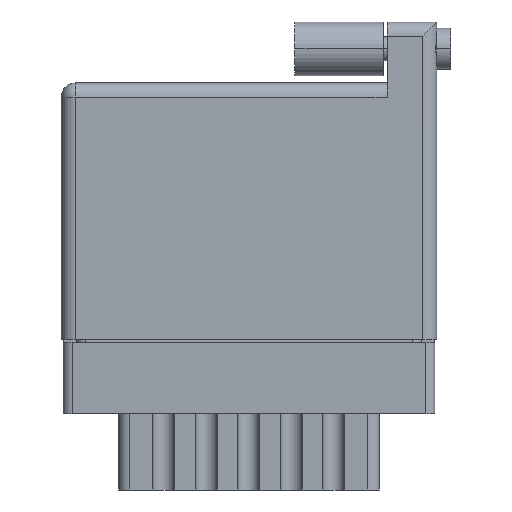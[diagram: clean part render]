
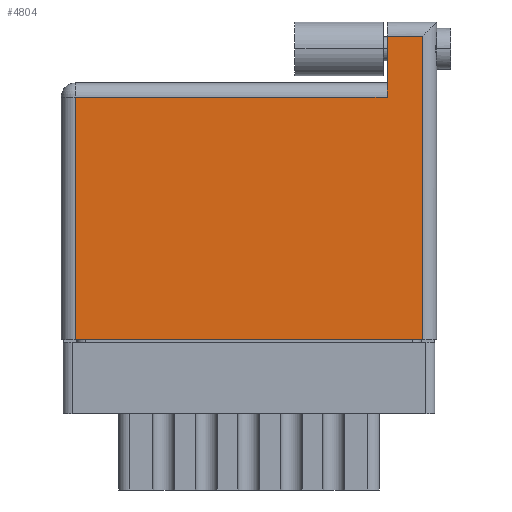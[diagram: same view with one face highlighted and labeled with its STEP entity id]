
A CAD part, front view. The second image highlights one B-rep face of the part: STEP entity #4804.
In plain terms, the highlighted face is planar.
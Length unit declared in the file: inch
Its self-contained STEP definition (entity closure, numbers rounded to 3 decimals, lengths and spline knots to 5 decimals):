
#594 = VECTOR ( 'NONE', #10157, 39.37008 ) ;
#1062 = EDGE_CURVE ( 'NONE', #4024, #21036, #1137, .T. ) ;
#1137 = LINE ( 'NONE', #23195, #19024 ) ;
#1382 = VECTOR ( 'NONE', #20869, 39.37008 ) ;
#2730 = LINE ( 'NONE', #8663, #12958 ) ;
#3134 = DIRECTION ( 'NONE',  ( 0., 1., 0. ) ) ;
#4024 = VERTEX_POINT ( 'NONE', #18156 ) ;
#4469 = ORIENTED_EDGE ( 'NONE', *, *, #6745, .T. ) ;
#4804 = ADVANCED_FACE ( 'NONE', ( #18088 ), #14244, .F. ) ;
#4963 = VERTEX_POINT ( 'NONE', #18463 ) ;
#5287 = DIRECTION ( 'NONE',  ( 1., 0., 0. ) ) ;
#5541 = CARTESIAN_POINT ( 'NONE',  ( 0., 0., 0. ) ) ;
#5773 = VECTOR ( 'NONE', #5287, 39.37008 ) ;
#6048 = VECTOR ( 'NONE', #17000, 39.37008 ) ;
#6083 = EDGE_CURVE ( 'NONE', #23491, #4024, #9254, .T. ) ;
#6106 = ORIENTED_EDGE ( 'NONE', *, *, #12518, .T. ) ;
#6311 = DIRECTION ( 'NONE',  ( -1., 0., 0. ) ) ;
#6745 = EDGE_CURVE ( 'NONE', #4963, #23491, #2730, .T. ) ;
#6818 = EDGE_LOOP ( 'NONE', ( #10099, #18596, #6106, #24164, #17749, #4469 ) ) ;
#7009 = CARTESIAN_POINT ( 'NONE',  ( 1.15, 1.12, 0. ) ) ;
#8663 = CARTESIAN_POINT ( 'NONE',  ( 0.05, 0., 0. ) ) ;
#8817 = CARTESIAN_POINT ( 'NONE',  ( 0., 1.07, 0. ) ) ;
#9254 = LINE ( 'NONE', #5541, #5773 ) ;
#10099 = ORIENTED_EDGE ( 'NONE', *, *, #6083, .T. ) ;
#10157 = DIRECTION ( 'NONE',  ( -1., 0., 0. ) ) ;
#11992 = VERTEX_POINT ( 'NONE', #20479 ) ;
#12518 = EDGE_CURVE ( 'NONE', #21036, #11992, #18841, .T. ) ;
#12815 = LINE ( 'NONE', #7009, #1382 ) ;
#12958 = VECTOR ( 'NONE', #14736, 39.37008 ) ;
#13113 = CARTESIAN_POINT ( 'NONE',  ( 1.15, 0.856, 0. ) ) ;
#13225 = CARTESIAN_POINT ( 'NONE',  ( 0.05, 0., 0. ) ) ;
#13592 = EDGE_CURVE ( 'NONE', #20471, #4963, #24172, .T. ) ;
#14244 = PLANE ( 'NONE',  #19278 ) ;
#14736 = DIRECTION ( 'NONE',  ( 0., -1., 0. ) ) ;
#15073 = EDGE_CURVE ( 'NONE', #11992, #20471, #12815, .T. ) ;
#15841 = DIRECTION ( 'NONE',  ( 0., 0., -1. ) ) ;
#15860 = CARTESIAN_POINT ( 'NONE',  ( 0., 0.856, 0. ) ) ;
#16344 = CARTESIAN_POINT ( 'NONE',  ( 0., 0.906, 0. ) ) ;
#17000 = DIRECTION ( 'NONE',  ( -1., 0., 0. ) ) ;
#17749 = ORIENTED_EDGE ( 'NONE', *, *, #13592, .T. ) ;
#18088 = FACE_OUTER_BOUND ( 'NONE', #6818, .T. ) ;
#18156 = CARTESIAN_POINT ( 'NONE',  ( 1.275, 0., 0. ) ) ;
#18463 = CARTESIAN_POINT ( 'NONE',  ( 0.05, 0.856, 0. ) ) ;
#18596 = ORIENTED_EDGE ( 'NONE', *, *, #1062, .T. ) ;
#18841 = LINE ( 'NONE', #8817, #6048 ) ;
#19024 = VECTOR ( 'NONE', #3134, 39.37008 ) ;
#19278 = AXIS2_PLACEMENT_3D ( 'NONE', #16344, #15841, #6311 ) ;
#20471 = VERTEX_POINT ( 'NONE', #13113 ) ;
#20479 = CARTESIAN_POINT ( 'NONE',  ( 1.15, 1.07, 0. ) ) ;
#20869 = DIRECTION ( 'NONE',  ( 0., -1., 0. ) ) ;
#21036 = VERTEX_POINT ( 'NONE', #23658 ) ;
#23195 = CARTESIAN_POINT ( 'NONE',  ( 1.275, 1.12, 0. ) ) ;
#23491 = VERTEX_POINT ( 'NONE', #13225 ) ;
#23658 = CARTESIAN_POINT ( 'NONE',  ( 1.275, 1.07, 0. ) ) ;
#24164 = ORIENTED_EDGE ( 'NONE', *, *, #15073, .T. ) ;
#24172 = LINE ( 'NONE', #15860, #594 ) ;
